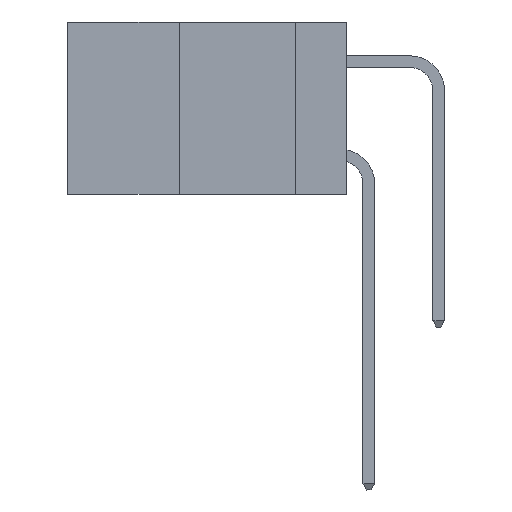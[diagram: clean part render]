
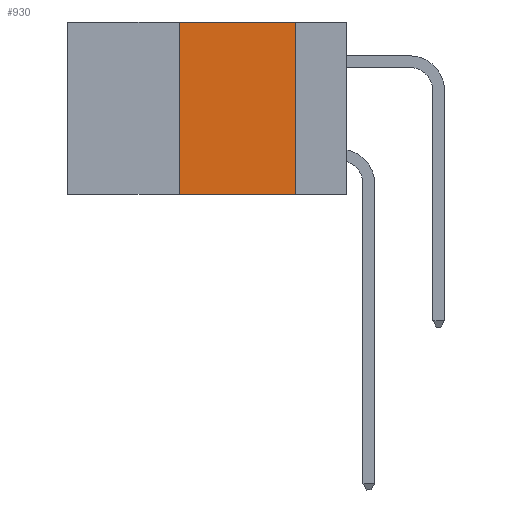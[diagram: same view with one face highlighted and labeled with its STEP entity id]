
A CAD part, left-side view. The second image highlights one B-rep face of the part: STEP entity #930.
In plain terms, the highlighted planar face has unit normal (-1, 0, 0).
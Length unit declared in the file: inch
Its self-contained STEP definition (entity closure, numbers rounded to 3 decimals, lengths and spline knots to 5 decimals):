
#154 = ORIENTED_EDGE ( 'NONE', *, *, #1364, .F. ) ;
#364 = CARTESIAN_POINT ( 'NONE',  ( 0., 0.11, 0. ) ) ;
#930 = ADVANCED_FACE ( 'NONE', ( #7279 ), #7922, .F. ) ;
#1219 = LINE ( 'NONE', #11114, #10805 ) ;
#1364 = EDGE_CURVE ( 'NONE', #10789, #2261, #7270, .T. ) ;
#1683 = ORIENTED_EDGE ( 'NONE', *, *, #11984, .F. ) ;
#1919 = ORIENTED_EDGE ( 'NONE', *, *, #9012, .F. ) ;
#2261 = VERTEX_POINT ( 'NONE', #5341 ) ;
#2289 = ORIENTED_EDGE ( 'NONE', *, *, #10735, .T. ) ;
#2297 = VECTOR ( 'NONE', #5429, 39.37008 ) ;
#2731 = CARTESIAN_POINT ( 'NONE',  ( 0., 0.6, -0.37 ) ) ;
#2814 = CARTESIAN_POINT ( 'NONE',  ( 0., 0.36, -0.37 ) ) ;
#3297 = VERTEX_POINT ( 'NONE', #10662 ) ;
#3717 = DIRECTION ( 'NONE',  ( 0., -1., 0. ) ) ;
#4044 = CARTESIAN_POINT ( 'NONE',  ( 0., 0.11, 0. ) ) ;
#4550 = EDGE_LOOP ( 'NONE', ( #1919, #1683, #154, #2289 ) ) ;
#5341 = CARTESIAN_POINT ( 'NONE',  ( 0., 0.36, 0. ) ) ;
#5429 = DIRECTION ( 'NONE',  ( 0., 0., 1. ) ) ;
#5673 = AXIS2_PLACEMENT_3D ( 'NONE', #9804, #9793, #8848 ) ;
#5722 = VECTOR ( 'NONE', #7013, 39.37008 ) ;
#6011 = LINE ( 'NONE', #364, #5722 ) ;
#6551 = VECTOR ( 'NONE', #3717, 39.37008 ) ;
#6768 = CARTESIAN_POINT ( 'NONE',  ( 0., 0.36, 0. ) ) ;
#7013 = DIRECTION ( 'NONE',  ( 0., 0., -1. ) ) ;
#7270 = LINE ( 'NONE', #6768, #2297 ) ;
#7279 = FACE_OUTER_BOUND ( 'NONE', #4550, .T. ) ;
#7922 = PLANE ( 'NONE',  #5673 ) ;
#8838 = VERTEX_POINT ( 'NONE', #4044 ) ;
#8848 = DIRECTION ( 'NONE',  ( 0., 0., -1. ) ) ;
#9012 = EDGE_CURVE ( 'NONE', #8838, #3297, #6011, .T. ) ;
#9356 = DIRECTION ( 'NONE',  ( 0., -1., 0. ) ) ;
#9793 = DIRECTION ( 'NONE',  ( 1., 0., 0. ) ) ;
#9804 = CARTESIAN_POINT ( 'NONE',  ( 0., 0.6, 0. ) ) ;
#10662 = CARTESIAN_POINT ( 'NONE',  ( 0., 0.11, -0.37 ) ) ;
#10735 = EDGE_CURVE ( 'NONE', #10789, #3297, #11381, .T. ) ;
#10789 = VERTEX_POINT ( 'NONE', #2814 ) ;
#10805 = VECTOR ( 'NONE', #9356, 39.37008 ) ;
#11114 = CARTESIAN_POINT ( 'NONE',  ( 0., 0.6, 0. ) ) ;
#11381 = LINE ( 'NONE', #2731, #6551 ) ;
#11984 = EDGE_CURVE ( 'NONE', #2261, #8838, #1219, .T. ) ;
